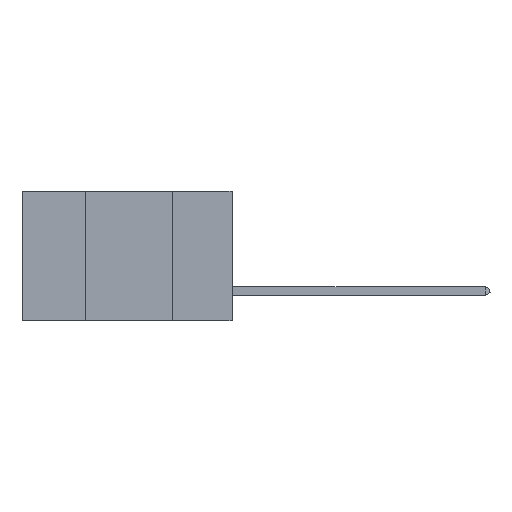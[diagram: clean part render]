
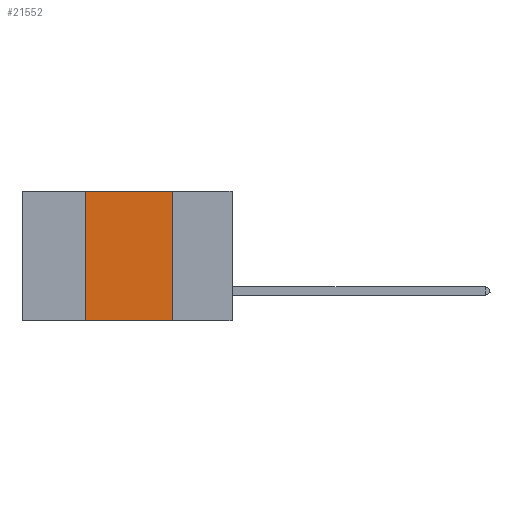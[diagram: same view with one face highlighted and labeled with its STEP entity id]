
A CAD part, left-side view. The second image highlights one B-rep face of the part: STEP entity #21552.
In plain terms, the highlighted planar face has unit normal (-1, 0, 0).
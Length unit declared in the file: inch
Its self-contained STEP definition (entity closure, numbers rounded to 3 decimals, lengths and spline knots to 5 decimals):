
#429 = EDGE_LOOP ( 'NONE', ( #29774, #5582, #5513, #15198 ) ) ;
#1555 = DIRECTION ( 'NONE',  ( 0., 0., -1. ) ) ;
#1859 = CARTESIAN_POINT ( 'NONE',  ( 0., 0.6, 0. ) ) ;
#3525 = VERTEX_POINT ( 'NONE', #16788 ) ;
#3597 = CARTESIAN_POINT ( 'NONE',  ( 0., 0.42, 0. ) ) ;
#3672 = FACE_OUTER_BOUND ( 'NONE', #429, .T. ) ;
#3803 = CARTESIAN_POINT ( 'NONE',  ( 0., 0.6, 0. ) ) ;
#3985 = EDGE_CURVE ( 'NONE', #13502, #29418, #13821, .T. ) ;
#5513 = ORIENTED_EDGE ( 'NONE', *, *, #15445, .F. ) ;
#5582 = ORIENTED_EDGE ( 'NONE', *, *, #8920, .F. ) ;
#8733 = CARTESIAN_POINT ( 'NONE',  ( 0., 0.42, -0.37 ) ) ;
#8920 = EDGE_CURVE ( 'NONE', #3525, #22167, #32703, .T. ) ;
#9271 = CARTESIAN_POINT ( 'NONE',  ( 0., 0.17, 0. ) ) ;
#11774 = DIRECTION ( 'NONE',  ( 0., -1., 0. ) ) ;
#13502 = VERTEX_POINT ( 'NONE', #8733 ) ;
#13643 = VECTOR ( 'NONE', #14710, 39.37008 ) ;
#13821 = LINE ( 'NONE', #25117, #30120 ) ;
#14710 = DIRECTION ( 'NONE',  ( 0., 0., 1. ) ) ;
#15198 = ORIENTED_EDGE ( 'NONE', *, *, #3985, .T. ) ;
#15445 = EDGE_CURVE ( 'NONE', #13502, #3525, #37689, .T. ) ;
#16788 = CARTESIAN_POINT ( 'NONE',  ( 0., 0.42, 0. ) ) ;
#18406 = DIRECTION ( 'NONE',  ( 0., -1., 0. ) ) ;
#21552 = ADVANCED_FACE ( 'NONE', ( #3672 ), #41095, .F. ) ;
#22167 = VERTEX_POINT ( 'NONE', #32992 ) ;
#24520 = VECTOR ( 'NONE', #27298, 39.37008 ) ;
#25117 = CARTESIAN_POINT ( 'NONE',  ( 0., 0.6, -0.37 ) ) ;
#26002 = VECTOR ( 'NONE', #11774, 39.37008 ) ;
#27051 = DIRECTION ( 'NONE',  ( 1., 0., 0. ) ) ;
#27298 = DIRECTION ( 'NONE',  ( 0., 0., -1. ) ) ;
#29418 = VERTEX_POINT ( 'NONE', #31421 ) ;
#29774 = ORIENTED_EDGE ( 'NONE', *, *, #45735, .F. ) ;
#30120 = VECTOR ( 'NONE', #18406, 39.37008 ) ;
#31421 = CARTESIAN_POINT ( 'NONE',  ( 0., 0.17, -0.37 ) ) ;
#32703 = LINE ( 'NONE', #3803, #26002 ) ;
#32992 = CARTESIAN_POINT ( 'NONE',  ( 0., 0.17, 0. ) ) ;
#37689 = LINE ( 'NONE', #3597, #13643 ) ;
#38367 = AXIS2_PLACEMENT_3D ( 'NONE', #1859, #27051, #1555 ) ;
#38508 = LINE ( 'NONE', #9271, #24520 ) ;
#41095 = PLANE ( 'NONE',  #38367 ) ;
#45735 = EDGE_CURVE ( 'NONE', #22167, #29418, #38508, .T. ) ;
